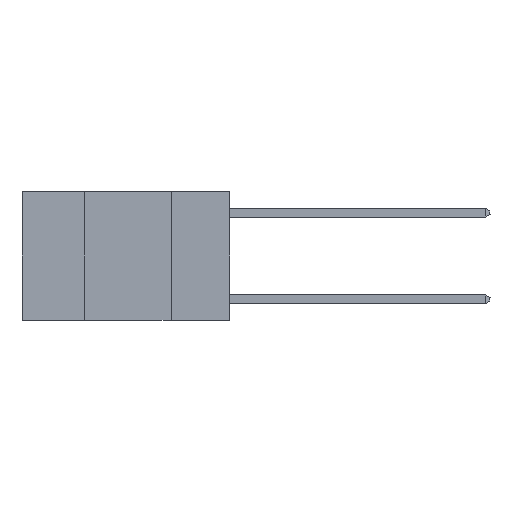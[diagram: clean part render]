
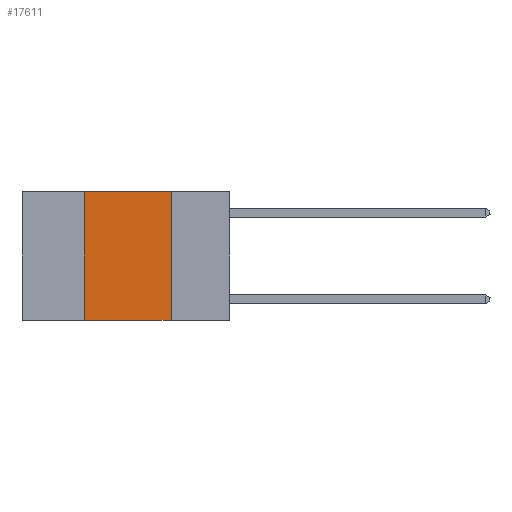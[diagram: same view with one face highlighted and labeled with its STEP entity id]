
A CAD part, left-side view. The second image highlights one B-rep face of the part: STEP entity #17611.
In plain terms, the highlighted planar face has unit normal (-1, 0, 0).
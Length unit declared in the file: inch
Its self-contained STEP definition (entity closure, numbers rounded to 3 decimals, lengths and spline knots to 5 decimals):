
#525 = CARTESIAN_POINT ( 'NONE',  ( 0., 0.42, 0. ) ) ;
#527 = ORIENTED_EDGE ( 'NONE', *, *, #21184, .F. ) ;
#530 = VECTOR ( 'NONE', #4167, 39.37008 ) ;
#2793 = DIRECTION ( 'NONE',  ( 0., 0., -1. ) ) ;
#3338 = CARTESIAN_POINT ( 'NONE',  ( 0., 0.42, -0.37 ) ) ;
#3519 = CARTESIAN_POINT ( 'NONE',  ( 0., 0.6, -0.37 ) ) ;
#3715 = VECTOR ( 'NONE', #11332, 39.37008 ) ;
#4167 = DIRECTION ( 'NONE',  ( 0., -1., 0. ) ) ;
#5256 = VECTOR ( 'NONE', #15593, 39.37008 ) ;
#5502 = LINE ( 'NONE', #15175, #530 ) ;
#5779 = LINE ( 'NONE', #525, #3715 ) ;
#6561 = CARTESIAN_POINT ( 'NONE',  ( 0., 0.6, 0. ) ) ;
#6650 = CARTESIAN_POINT ( 'NONE',  ( 0., 0.17, 0. ) ) ;
#6845 = EDGE_CURVE ( 'NONE', #12327, #10682, #5502, .T. ) ;
#8132 = PLANE ( 'NONE',  #21779 ) ;
#8590 = EDGE_CURVE ( 'NONE', #10081, #13829, #10565, .T. ) ;
#9025 = ORIENTED_EDGE ( 'NONE', *, *, #8590, .T. ) ;
#9825 = FACE_OUTER_BOUND ( 'NONE', #16891, .T. ) ;
#10081 = VERTEX_POINT ( 'NONE', #3338 ) ;
#10565 = LINE ( 'NONE', #3519, #19814 ) ;
#10682 = VERTEX_POINT ( 'NONE', #11985 ) ;
#11332 = DIRECTION ( 'NONE',  ( 0., 0., 1. ) ) ;
#11985 = CARTESIAN_POINT ( 'NONE',  ( 0., 0.17, 0. ) ) ;
#12090 = LINE ( 'NONE', #6650, #5256 ) ;
#12327 = VERTEX_POINT ( 'NONE', #19957 ) ;
#13829 = VERTEX_POINT ( 'NONE', #16221 ) ;
#13920 = DIRECTION ( 'NONE',  ( 1., 0., 0. ) ) ;
#15133 = ORIENTED_EDGE ( 'NONE', *, *, #19440, .F. ) ;
#15175 = CARTESIAN_POINT ( 'NONE',  ( 0., 0.6, 0. ) ) ;
#15593 = DIRECTION ( 'NONE',  ( 0., 0., -1. ) ) ;
#16221 = CARTESIAN_POINT ( 'NONE',  ( 0., 0.17, -0.37 ) ) ;
#16891 = EDGE_LOOP ( 'NONE', ( #15133, #20822, #527, #9025 ) ) ;
#17611 = ADVANCED_FACE ( 'NONE', ( #9825 ), #8132, .F. ) ;
#19310 = DIRECTION ( 'NONE',  ( 0., -1., 0. ) ) ;
#19440 = EDGE_CURVE ( 'NONE', #10682, #13829, #12090, .T. ) ;
#19814 = VECTOR ( 'NONE', #19310, 39.37008 ) ;
#19957 = CARTESIAN_POINT ( 'NONE',  ( 0., 0.42, 0. ) ) ;
#20822 = ORIENTED_EDGE ( 'NONE', *, *, #6845, .F. ) ;
#21184 = EDGE_CURVE ( 'NONE', #10081, #12327, #5779, .T. ) ;
#21779 = AXIS2_PLACEMENT_3D ( 'NONE', #6561, #13920, #2793 ) ;
